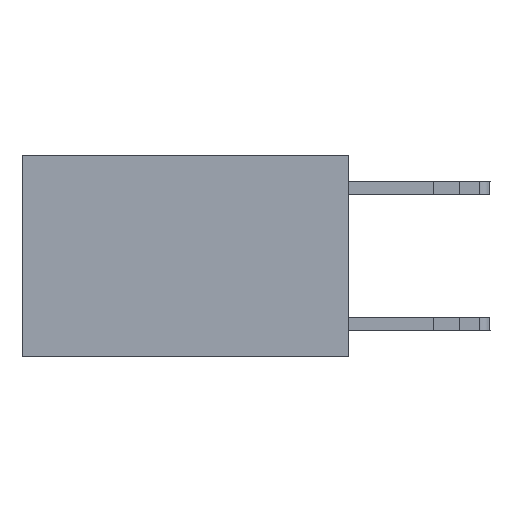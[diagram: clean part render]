
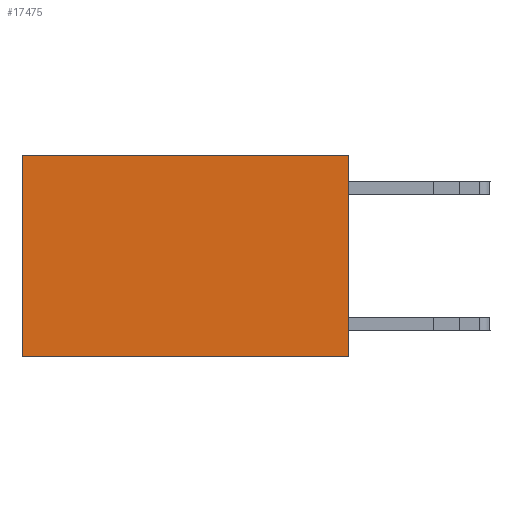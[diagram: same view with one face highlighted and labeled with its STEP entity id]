
A CAD part, left-side view. The second image highlights one B-rep face of the part: STEP entity #17475.
In plain terms, the highlighted planar face has unit normal (-1, 0, 0).
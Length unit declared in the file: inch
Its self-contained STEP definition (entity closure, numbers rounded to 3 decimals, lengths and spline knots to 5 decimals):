
#1232 = VECTOR ( 'NONE', #15088, 39.37008 ) ;
#2501 = AXIS2_PLACEMENT_3D ( 'NONE', #27841, #18340, #4663 ) ;
#3515 = EDGE_CURVE ( 'NONE', #22807, #14243, #7313, .T. ) ;
#3578 = CARTESIAN_POINT ( 'NONE',  ( 0.2625, 0.6, -0.37 ) ) ;
#4393 = CARTESIAN_POINT ( 'NONE',  ( 0.2625, 0., 0. ) ) ;
#4663 = DIRECTION ( 'NONE',  ( 0., 0., -1. ) ) ;
#7269 = CARTESIAN_POINT ( 'NONE',  ( 0.2625, 0., 0. ) ) ;
#7313 = LINE ( 'NONE', #23403, #21114 ) ;
#8506 = VERTEX_POINT ( 'NONE', #12381 ) ;
#8750 = DIRECTION ( 'NONE',  ( 0., 1., 0. ) ) ;
#9517 = DIRECTION ( 'NONE',  ( 0., 0., -1. ) ) ;
#9617 = ORIENTED_EDGE ( 'NONE', *, *, #3515, .F. ) ;
#11305 = VECTOR ( 'NONE', #8750, 39.37008 ) ;
#11364 = DIRECTION ( 'NONE',  ( 0., 1., 0. ) ) ;
#12381 = CARTESIAN_POINT ( 'NONE',  ( 0.2625, 0., 0. ) ) ;
#14243 = VERTEX_POINT ( 'NONE', #3578 ) ;
#15088 = DIRECTION ( 'NONE',  ( 0., 0., -1. ) ) ;
#16795 = CARTESIAN_POINT ( 'NONE',  ( 0.2625, 0.6, 0. ) ) ;
#17081 = EDGE_CURVE ( 'NONE', #8506, #22807, #25311, .T. ) ;
#17325 = ORIENTED_EDGE ( 'NONE', *, *, #17081, .F. ) ;
#17475 = ADVANCED_FACE ( 'NONE', ( #23880 ), #25426, .F. ) ;
#18340 = DIRECTION ( 'NONE',  ( 1., 0., 0. ) ) ;
#18622 = ORIENTED_EDGE ( 'NONE', *, *, #21728, .T. ) ;
#19650 = VERTEX_POINT ( 'NONE', #16795 ) ;
#20707 = VECTOR ( 'NONE', #9517, 39.37008 ) ;
#21114 = VECTOR ( 'NONE', #11364, 39.37008 ) ;
#21130 = CARTESIAN_POINT ( 'NONE',  ( 0.2625, 0., -0.37 ) ) ;
#21551 = EDGE_CURVE ( 'NONE', #19650, #14243, #24131, .T. ) ;
#21728 = EDGE_CURVE ( 'NONE', #8506, #19650, #24848, .T. ) ;
#22807 = VERTEX_POINT ( 'NONE', #21130 ) ;
#23403 = CARTESIAN_POINT ( 'NONE',  ( 0.2625, 0., -0.37 ) ) ;
#23880 = FACE_OUTER_BOUND ( 'NONE', #25132, .T. ) ;
#24131 = LINE ( 'NONE', #24426, #1232 ) ;
#24370 = ORIENTED_EDGE ( 'NONE', *, *, #21551, .T. ) ;
#24426 = CARTESIAN_POINT ( 'NONE',  ( 0.2625, 0.6, 0. ) ) ;
#24848 = LINE ( 'NONE', #4393, #11305 ) ;
#25132 = EDGE_LOOP ( 'NONE', ( #24370, #9617, #17325, #18622 ) ) ;
#25311 = LINE ( 'NONE', #7269, #20707 ) ;
#25426 = PLANE ( 'NONE',  #2501 ) ;
#27841 = CARTESIAN_POINT ( 'NONE',  ( 0.2625, 0., 0. ) ) ;
